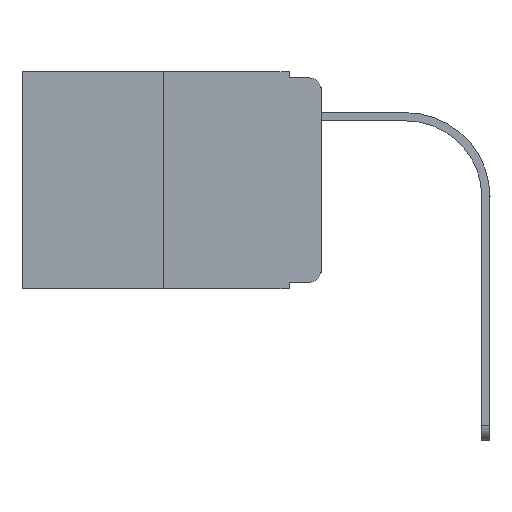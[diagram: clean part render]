
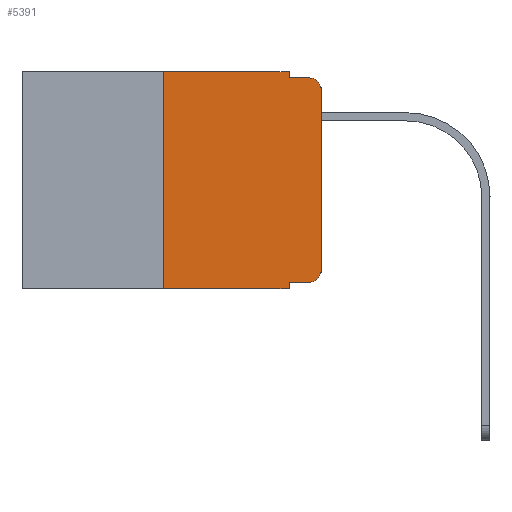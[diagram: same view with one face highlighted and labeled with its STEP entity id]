
A CAD part, left-side view. The second image highlights one B-rep face of the part: STEP entity #5391.
In plain terms, the highlighted planar face has unit normal (-1, 0, 0).
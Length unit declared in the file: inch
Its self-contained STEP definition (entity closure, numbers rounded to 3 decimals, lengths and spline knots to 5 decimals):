
#64 = VECTOR ( 'NONE', #15011, 39.37008 ) ;
#99 = LINE ( 'NONE', #6762, #395 ) ;
#233 = CARTESIAN_POINT ( 'NONE',  ( 0., 0.051, -0.343 ) ) ;
#395 = VECTOR ( 'NONE', #9354, 39.37008 ) ;
#429 = ORIENTED_EDGE ( 'NONE', *, *, #8038, .T. ) ;
#529 = DIRECTION ( 'NONE',  ( 0., 0., -1. ) ) ;
#915 = VECTOR ( 'NONE', #529, 39.37008 ) ;
#1128 = LINE ( 'NONE', #16245, #17124 ) ;
#1145 = PLANE ( 'NONE',  #4102 ) ;
#1261 = VECTOR ( 'NONE', #3220, 39.37008 ) ;
#1286 = CARTESIAN_POINT ( 'NONE',  ( 0., 0.25, 0. ) ) ;
#1371 = ORIENTED_EDGE ( 'NONE', *, *, #6933, .T. ) ;
#1543 = LINE ( 'NONE', #12830, #1261 ) ;
#3020 = DIRECTION ( 'NONE',  ( 0., 0., -1. ) ) ;
#3183 = CARTESIAN_POINT ( 'NONE',  ( 0., 0.051, 0. ) ) ;
#3220 = DIRECTION ( 'NONE',  ( 0., -1., 0. ) ) ;
#3294 = CARTESIAN_POINT ( 'NONE',  ( 0., 0.473, -0.343 ) ) ;
#3356 = DIRECTION ( 'NONE',  ( 0., 0., -1. ) ) ;
#3472 = DIRECTION ( 'NONE',  ( 0., -1., 0. ) ) ;
#3666 = ORIENTED_EDGE ( 'NONE', *, *, #6728, .T. ) ;
#4102 = AXIS2_PLACEMENT_3D ( 'NONE', #17245, #6648, #11758 ) ;
#4520 = CIRCLE ( 'NONE', #11387, 0.02 ) ;
#4752 = CARTESIAN_POINT ( 'NONE',  ( 0., 0.051, -0.01 ) ) ;
#5187 = EDGE_CURVE ( 'NONE', #10673, #9430, #10080, .T. ) ;
#5365 = ORIENTED_EDGE ( 'NONE', *, *, #8034, .F. ) ;
#5391 = ADVANCED_FACE ( 'NONE', ( #13464 ), #1145, .F. ) ;
#5396 = VERTEX_POINT ( 'NONE', #5754 ) ;
#5465 = EDGE_CURVE ( 'NONE', #6900, #9661, #12299, .T. ) ;
#5754 = CARTESIAN_POINT ( 'NONE',  ( 0., 0.051, 0. ) ) ;
#6627 = CARTESIAN_POINT ( 'NONE',  ( 0., 0.02, -0.313 ) ) ;
#6648 = DIRECTION ( 'NONE',  ( 1., 0., 0. ) ) ;
#6659 = VECTOR ( 'NONE', #11518, 39.37008 ) ;
#6728 = EDGE_CURVE ( 'NONE', #13597, #11377, #99, .T. ) ;
#6762 = CARTESIAN_POINT ( 'NONE',  ( 0., 0., 0. ) ) ;
#6900 = VERTEX_POINT ( 'NONE', #4752 ) ;
#6933 = EDGE_CURVE ( 'NONE', #10673, #12072, #1543, .T. ) ;
#7152 = DIRECTION ( 'NONE',  ( -1., 0., 0. ) ) ;
#7210 = LINE ( 'NONE', #10007, #6659 ) ;
#7254 = EDGE_LOOP ( 'NONE', ( #3666, #14567, #15865, #13224, #5365, #12697, #16038, #14076, #1371, #429 ) ) ;
#7875 = DIRECTION ( 'NONE',  ( -1., 0., 0. ) ) ;
#7878 = VECTOR ( 'NONE', #3472, 39.37008 ) ;
#8034 = EDGE_CURVE ( 'NONE', #15567, #5396, #1128, .T. ) ;
#8038 = EDGE_CURVE ( 'NONE', #12072, #13597, #14557, .T. ) ;
#8260 = CARTESIAN_POINT ( 'NONE',  ( 0., 0.051, -0.01 ) ) ;
#8281 = EDGE_CURVE ( 'NONE', #11377, #9661, #4520, .T. ) ;
#8726 = CARTESIAN_POINT ( 'NONE',  ( 0., 0.051, 0. ) ) ;
#8927 = CARTESIAN_POINT ( 'NONE',  ( 0., 0., -0.03 ) ) ;
#9354 = DIRECTION ( 'NONE',  ( 0., 0., 1. ) ) ;
#9430 = VERTEX_POINT ( 'NONE', #233 ) ;
#9661 = VERTEX_POINT ( 'NONE', #16946 ) ;
#10007 = CARTESIAN_POINT ( 'NONE',  ( 0., 0.25, 0. ) ) ;
#10080 = LINE ( 'NONE', #8726, #915 ) ;
#10393 = LINE ( 'NONE', #3294, #7878 ) ;
#10673 = VERTEX_POINT ( 'NONE', #12307 ) ;
#11377 = VERTEX_POINT ( 'NONE', #8927 ) ;
#11387 = AXIS2_PLACEMENT_3D ( 'NONE', #15512, #7152, #3020 ) ;
#11518 = DIRECTION ( 'NONE',  ( 0., 0., 1. ) ) ;
#11710 = CARTESIAN_POINT ( 'NONE',  ( 0., 0.25, -0.343 ) ) ;
#11758 = DIRECTION ( 'NONE',  ( 0., 0., -1. ) ) ;
#12072 = VERTEX_POINT ( 'NONE', #15070 ) ;
#12280 = EDGE_CURVE ( 'NONE', #5396, #6900, #16933, .T. ) ;
#12299 = LINE ( 'NONE', #8260, #64 ) ;
#12307 = CARTESIAN_POINT ( 'NONE',  ( 0., 0.051, -0.333 ) ) ;
#12376 = VERTEX_POINT ( 'NONE', #11710 ) ;
#12644 = EDGE_CURVE ( 'NONE', #12376, #15567, #7210, .T. ) ;
#12675 = VECTOR ( 'NONE', #3356, 39.37008 ) ;
#12697 = ORIENTED_EDGE ( 'NONE', *, *, #12644, .F. ) ;
#12830 = CARTESIAN_POINT ( 'NONE',  ( 0., 0.051, -0.333 ) ) ;
#13224 = ORIENTED_EDGE ( 'NONE', *, *, #12280, .F. ) ;
#13356 = DIRECTION ( 'NONE',  ( 0., 0., -1. ) ) ;
#13464 = FACE_OUTER_BOUND ( 'NONE', #7254, .T. ) ;
#13597 = VERTEX_POINT ( 'NONE', #15354 ) ;
#13653 = EDGE_CURVE ( 'NONE', #12376, #9430, #10393, .T. ) ;
#14076 = ORIENTED_EDGE ( 'NONE', *, *, #5187, .F. ) ;
#14265 = AXIS2_PLACEMENT_3D ( 'NONE', #6627, #7875, #13356 ) ;
#14536 = DIRECTION ( 'NONE',  ( 0., -1., 0. ) ) ;
#14557 = CIRCLE ( 'NONE', #14265, 0.02 ) ;
#14567 = ORIENTED_EDGE ( 'NONE', *, *, #8281, .T. ) ;
#15011 = DIRECTION ( 'NONE',  ( 0., -1., 0. ) ) ;
#15070 = CARTESIAN_POINT ( 'NONE',  ( 0., 0.02, -0.333 ) ) ;
#15354 = CARTESIAN_POINT ( 'NONE',  ( 0., 0., -0.313 ) ) ;
#15512 = CARTESIAN_POINT ( 'NONE',  ( 0., 0.02, -0.03 ) ) ;
#15567 = VERTEX_POINT ( 'NONE', #1286 ) ;
#15865 = ORIENTED_EDGE ( 'NONE', *, *, #5465, .F. ) ;
#16038 = ORIENTED_EDGE ( 'NONE', *, *, #13653, .T. ) ;
#16245 = CARTESIAN_POINT ( 'NONE',  ( 0., 0.473, 0. ) ) ;
#16933 = LINE ( 'NONE', #3183, #12675 ) ;
#16946 = CARTESIAN_POINT ( 'NONE',  ( 0., 0.02, -0.01 ) ) ;
#17124 = VECTOR ( 'NONE', #14536, 39.37008 ) ;
#17245 = CARTESIAN_POINT ( 'NONE',  ( 0., 0.473, 0. ) ) ;
